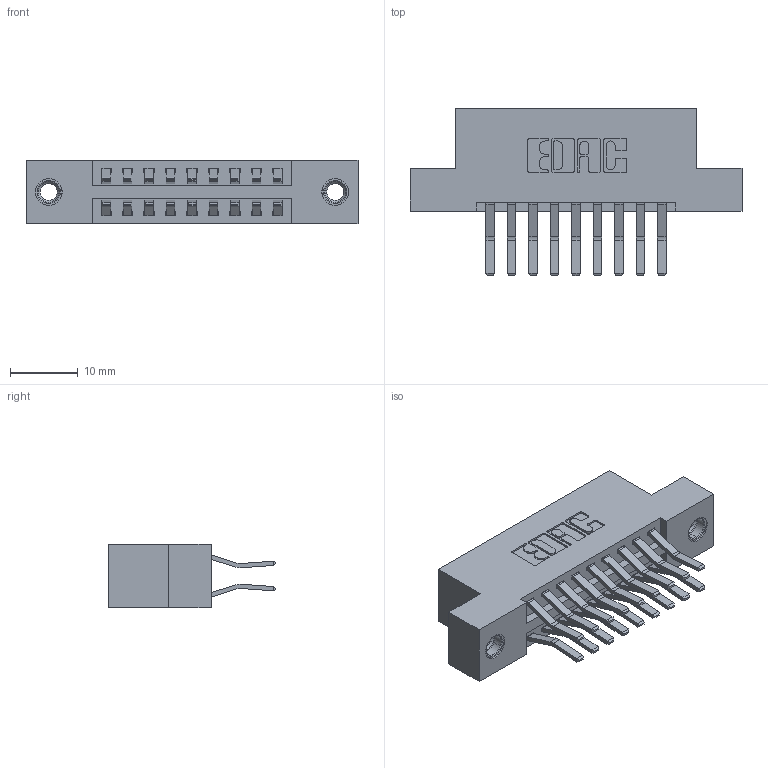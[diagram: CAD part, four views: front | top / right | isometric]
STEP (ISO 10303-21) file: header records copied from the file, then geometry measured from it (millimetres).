
FILE_DESCRIPTION (( 'STEP AP203' ), '1' );
FILE_NAME ('396-018-560-207.STEP', '2018-09-01T03:33:49', ( '' ), ( '' ), 'SwSTEP 2.0', 'SolidWorks 2016', '' );
FILE_SCHEMA (( 'CONFIG_CONTROL_DESIGN' ));
Length unit declared in the file: inch
Products named in the file (4): 346 Part_Flush Mounting Lugs - 0.156 Dia-TI; 345-292-001_560 Tail; 345-250-001_345-250-005-103; 396-018-560-207
Assembly tree (21 placements, depth 2):
  396-018-560-207
    346 Part_Flush Mounting Lugs - 0.156 Dia-TI
    345-292-001_560 Tail  x18
    345-250-001_345-250-005-103  x2
Bounding box: 49.15 x 24.78 x 9.4 mm (x, y, z)
Volume: 4640.8 mm3; surface area: 6208.9 mm2
Topology: 21 solids, 21 shells, 1154 faces, 3363 edges, 2210 vertices
Faces by surface type: plane 738, cylinder 400, cone 12, torus 4
Entity records: 11590 total; most frequent: CARTESIAN_POINT 1939, ORIENTED_EDGE 1866, DIRECTION 1791, EDGE_CURVE 933, LINE 741, VECTOR 741, VERTEX_POINT 616, AXIS2_PLACEMENT_3D 525
